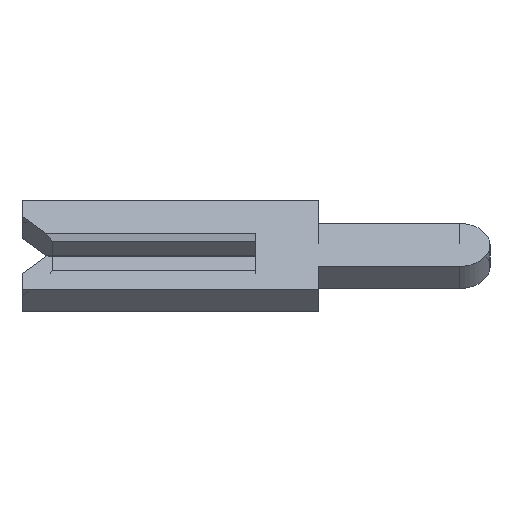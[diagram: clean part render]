
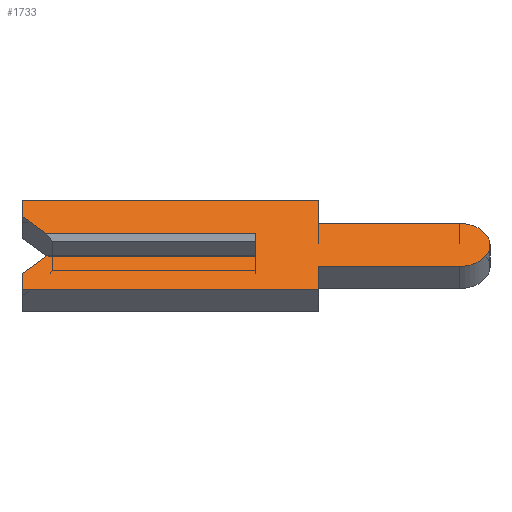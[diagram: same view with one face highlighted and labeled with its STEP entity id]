
A CAD part, left-side view. The second image highlights one B-rep face of the part: STEP entity #1733.
In plain terms, the highlighted face is planar.
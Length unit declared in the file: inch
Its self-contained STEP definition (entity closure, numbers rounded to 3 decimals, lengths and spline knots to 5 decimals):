
#27 = VECTOR ( 'NONE', #2829, 39.37008 ) ;
#31 = VECTOR ( 'NONE', #105, 39.37008 ) ;
#34 = ORIENTED_EDGE ( 'NONE', *, *, #1888, .F. ) ;
#54 = EDGE_CURVE ( 'NONE', #1884, #401, #1917, .T. ) ;
#76 = VERTEX_POINT ( 'NONE', #463 ) ;
#86 = LINE ( 'NONE', #2418, #445 ) ;
#105 = DIRECTION ( 'NONE',  ( 0., 0., -1. ) ) ;
#118 = CARTESIAN_POINT ( 'NONE',  ( -0.01, 0.15, 0.01 ) ) ;
#190 = ORIENTED_EDGE ( 'NONE', *, *, #1191, .T. ) ;
#203 = ORIENTED_EDGE ( 'NONE', *, *, #740, .F. ) ;
#235 = ORIENTED_EDGE ( 'NONE', *, *, #2253, .F. ) ;
#305 = VERTEX_POINT ( 'NONE', #483 ) ;
#317 = CARTESIAN_POINT ( 'NONE',  ( -0.01, 0.15, -0.04 ) ) ;
#361 = DIRECTION ( 'NONE',  ( 0., -1., 0. ) ) ;
#373 = DIRECTION ( 'NONE',  ( 1., 0., 0. ) ) ;
#381 = VERTEX_POINT ( 'NONE', #2295 ) ;
#401 = VERTEX_POINT ( 'NONE', #1810 ) ;
#445 = VECTOR ( 'NONE', #2313, 39.37008 ) ;
#463 = CARTESIAN_POINT ( 'NONE',  ( -0.01, -0.04, -0.0195 ) ) ;
#473 = CARTESIAN_POINT ( 'NONE',  ( -0.01, -0.1305, -0.01 ) ) ;
#481 = LINE ( 'NONE', #1503, #2178 ) ;
#482 = VECTOR ( 'NONE', #1150, 39.37008 ) ;
#483 = CARTESIAN_POINT ( 'NONE',  ( -0.01, 0., 0.01 ) ) ;
#490 = VECTOR ( 'NONE', #1471, 39.37008 ) ;
#516 = CARTESIAN_POINT ( 'NONE',  ( -0.01, -0.04, -0.0195 ) ) ;
#542 = LINE ( 'NONE', #576, #31 ) ;
#572 = ORIENTED_EDGE ( 'NONE', *, *, #2156, .F. ) ;
#576 = CARTESIAN_POINT ( 'NONE',  ( -0.01, -0.04, -0.04 ) ) ;
#589 = CARTESIAN_POINT ( 'NONE',  ( -0.01, -0.04, -0.04 ) ) ;
#619 = AXIS2_PLACEMENT_3D ( 'NONE', #1965, #1956, #1740 ) ;
#632 = CARTESIAN_POINT ( 'NONE',  ( -0.01, 0.15, 0.026 ) ) ;
#668 = CIRCLE ( 'NONE', #1921, 0.0195 ) ;
#675 = CARTESIAN_POINT ( 'NONE',  ( -0.01, -0.04, 0.04 ) ) ;
#681 = VERTEX_POINT ( 'NONE', #2786 ) ;
#685 = CARTESIAN_POINT ( 'NONE',  ( -0.01, 0.1305, 0.0065 ) ) ;
#709 = LINE ( 'NONE', #516, #1620 ) ;
#740 = EDGE_CURVE ( 'NONE', #1408, #76, #709, .T. ) ;
#804 = ORIENTED_EDGE ( 'NONE', *, *, #2610, .F. ) ;
#909 = CARTESIAN_POINT ( 'NONE',  ( -0.01, 0.15, 0.026 ) ) ;
#968 = LINE ( 'NONE', #473, #2533 ) ;
#1071 = CARTESIAN_POINT ( 'NONE',  ( -0.01, 0.15, -0.026 ) ) ;
#1078 = VECTOR ( 'NONE', #2868, 39.37008 ) ;
#1079 = VERTEX_POINT ( 'NONE', #1233 ) ;
#1083 = EDGE_CURVE ( 'NONE', #681, #305, #2579, .T. ) ;
#1084 = CARTESIAN_POINT ( 'NONE',  ( -0.01, 0.134, -0.01 ) ) ;
#1127 = ORIENTED_EDGE ( 'NONE', *, *, #2092, .F. ) ;
#1150 = DIRECTION ( 'NONE',  ( 0., 0., 1. ) ) ;
#1154 = LINE ( 'NONE', #1071, #1078 ) ;
#1191 = EDGE_CURVE ( 'NONE', #1203, #305, #1659, .T. ) ;
#1203 = VERTEX_POINT ( 'NONE', #2111 ) ;
#1233 = CARTESIAN_POINT ( 'NONE',  ( -0.01, 0.15, -0.026 ) ) ;
#1234 = ORIENTED_EDGE ( 'NONE', *, *, #1781, .F. ) ;
#1245 = ORIENTED_EDGE ( 'NONE', *, *, #1294, .F. ) ;
#1294 = EDGE_CURVE ( 'NONE', #1926, #381, #2213, .T. ) ;
#1309 = VERTEX_POINT ( 'NONE', #317 ) ;
#1408 = VERTEX_POINT ( 'NONE', #2377 ) ;
#1440 = EDGE_CURVE ( 'NONE', #76, #1552, #542, .T. ) ;
#1471 = DIRECTION ( 'NONE',  ( 0., 0., 1. ) ) ;
#1478 = CARTESIAN_POINT ( 'NONE',  ( -0.01, -0.04, 0.04 ) ) ;
#1479 = ORIENTED_EDGE ( 'NONE', *, *, #1540, .F. ) ;
#1503 = CARTESIAN_POINT ( 'NONE',  ( -0.01, 0.15, 0.04 ) ) ;
#1540 = EDGE_CURVE ( 'NONE', #2269, #1926, #2247, .T. ) ;
#1552 = VERTEX_POINT ( 'NONE', #589 ) ;
#1620 = VECTOR ( 'NONE', #2523, 39.37008 ) ;
#1659 = LINE ( 'NONE', #118, #27 ) ;
#1712 = DIRECTION ( 'NONE',  ( 0., 0., -1. ) ) ;
#1723 = VECTOR ( 'NONE', #2477, 39.37008 ) ;
#1731 = CARTESIAN_POINT ( 'NONE',  ( -0.01, 0.15, -0.04 ) ) ;
#1733 = ADVANCED_FACE ( 'NONE', ( #1783 ), #2657, .F. ) ;
#1740 = DIRECTION ( 'NONE',  ( 0., 0., -1. ) ) ;
#1781 = EDGE_CURVE ( 'NONE', #381, #1408, #668, .T. ) ;
#1783 = FACE_OUTER_BOUND ( 'NONE', #2133, .T. ) ;
#1810 = CARTESIAN_POINT ( 'NONE',  ( -0.01, 0.15, 0.04 ) ) ;
#1816 = LINE ( 'NONE', #1731, #2752 ) ;
#1884 = VERTEX_POINT ( 'NONE', #632 ) ;
#1888 = EDGE_CURVE ( 'NONE', #1079, #2626, #86, .T. ) ;
#1895 = DIRECTION ( 'NONE',  ( 0., -1., 0. ) ) ;
#1917 = LINE ( 'NONE', #909, #482 ) ;
#1921 = AXIS2_PLACEMENT_3D ( 'NONE', #1974, #373, #2664 ) ;
#1926 = VERTEX_POINT ( 'NONE', #2181 ) ;
#1943 = DIRECTION ( 'NONE',  ( 0., 1., 0. ) ) ;
#1956 = DIRECTION ( 'NONE',  ( 1., 0., 0. ) ) ;
#1965 = CARTESIAN_POINT ( 'NONE',  ( -0.01, -0.1305, 0. ) ) ;
#1974 = CARTESIAN_POINT ( 'NONE',  ( -0.01, -0.1305, 0. ) ) ;
#1994 = VECTOR ( 'NONE', #1895, 39.37008 ) ;
#2060 = DIRECTION ( 'NONE',  ( 0., -1., 0. ) ) ;
#2092 = EDGE_CURVE ( 'NONE', #1309, #1079, #1154, .T. ) ;
#2111 = CARTESIAN_POINT ( 'NONE',  ( -0.01, 0.134, 0.01 ) ) ;
#2132 = LINE ( 'NONE', #685, #1723 ) ;
#2133 = EDGE_LOOP ( 'NONE', ( #190, #2727, #2536, #34, #1127, #235, #2534, #203, #1234, #1245, #1479, #572, #2157, #804 ) ) ;
#2156 = EDGE_CURVE ( 'NONE', #401, #2269, #481, .T. ) ;
#2157 = ORIENTED_EDGE ( 'NONE', *, *, #54, .F. ) ;
#2178 = VECTOR ( 'NONE', #361, 39.37008 ) ;
#2181 = CARTESIAN_POINT ( 'NONE',  ( -0.01, -0.04, 0.0195 ) ) ;
#2213 = LINE ( 'NONE', #2813, #1994 ) ;
#2247 = LINE ( 'NONE', #1478, #2718 ) ;
#2253 = EDGE_CURVE ( 'NONE', #1552, #1309, #1816, .T. ) ;
#2269 = VERTEX_POINT ( 'NONE', #675 ) ;
#2295 = CARTESIAN_POINT ( 'NONE',  ( -0.01, -0.1305, 0.0195 ) ) ;
#2313 = DIRECTION ( 'NONE',  ( 0., -0.707, 0.707 ) ) ;
#2377 = CARTESIAN_POINT ( 'NONE',  ( -0.01, -0.1305, -0.0195 ) ) ;
#2418 = CARTESIAN_POINT ( 'NONE',  ( -0.01, 0.1305, -0.0065 ) ) ;
#2477 = DIRECTION ( 'NONE',  ( 0., 0.707, 0.707 ) ) ;
#2523 = DIRECTION ( 'NONE',  ( 0., 1., 0. ) ) ;
#2533 = VECTOR ( 'NONE', #2060, 39.37008 ) ;
#2534 = ORIENTED_EDGE ( 'NONE', *, *, #1440, .F. ) ;
#2536 = ORIENTED_EDGE ( 'NONE', *, *, #2759, .F. ) ;
#2579 = LINE ( 'NONE', #2821, #490 ) ;
#2610 = EDGE_CURVE ( 'NONE', #1203, #1884, #2132, .T. ) ;
#2626 = VERTEX_POINT ( 'NONE', #1084 ) ;
#2657 = PLANE ( 'NONE',  #619 ) ;
#2664 = DIRECTION ( 'NONE',  ( 0., 0., -1. ) ) ;
#2718 = VECTOR ( 'NONE', #1712, 39.37008 ) ;
#2727 = ORIENTED_EDGE ( 'NONE', *, *, #1083, .F. ) ;
#2752 = VECTOR ( 'NONE', #1943, 39.37008 ) ;
#2759 = EDGE_CURVE ( 'NONE', #2626, #681, #968, .T. ) ;
#2786 = CARTESIAN_POINT ( 'NONE',  ( -0.01, 0., -0.01 ) ) ;
#2813 = CARTESIAN_POINT ( 'NONE',  ( -0.01, -0.04, 0.0195 ) ) ;
#2821 = CARTESIAN_POINT ( 'NONE',  ( -0.01, 0., 0.0065 ) ) ;
#2829 = DIRECTION ( 'NONE',  ( 0., -1., 0. ) ) ;
#2868 = DIRECTION ( 'NONE',  ( 0., 0., 1. ) ) ;
